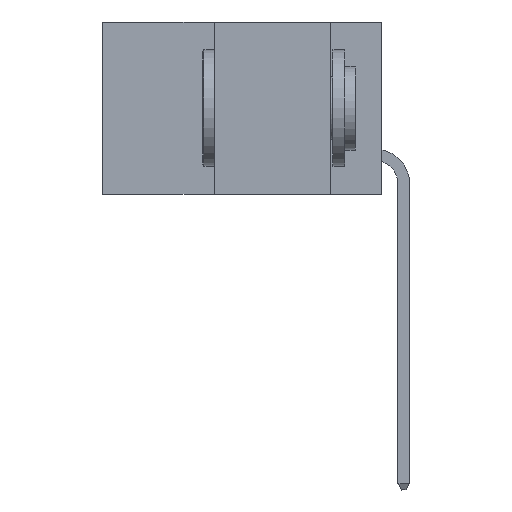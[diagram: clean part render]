
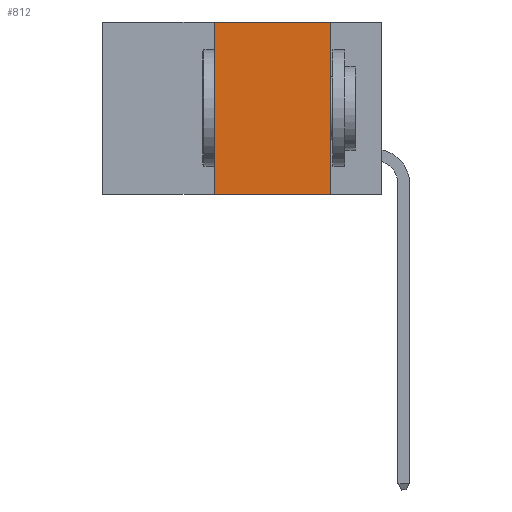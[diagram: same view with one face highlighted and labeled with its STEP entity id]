
A CAD part, left-side view. The second image highlights one B-rep face of the part: STEP entity #812.
In plain terms, the highlighted planar face has unit normal (-1, 0, 0).
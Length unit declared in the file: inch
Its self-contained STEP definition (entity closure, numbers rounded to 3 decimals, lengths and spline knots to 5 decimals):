
#757 = EDGE_CURVE ( 'NONE', #19557, #20888, #19914, .T. ) ;
#812 = ADVANCED_FACE ( 'NONE', ( #7493 ), #23499, .F. ) ;
#2360 = CARTESIAN_POINT ( 'NONE',  ( 0., 0.11, 0. ) ) ;
#3142 = EDGE_CURVE ( 'NONE', #5010, #19557, #9548, .T. ) ;
#3260 = CARTESIAN_POINT ( 'NONE',  ( 0., 0.6, 0. ) ) ;
#4250 = DIRECTION ( 'NONE',  ( 0., 0., -1. ) ) ;
#4699 = CARTESIAN_POINT ( 'NONE',  ( 0., 0.11, -0.37 ) ) ;
#5010 = VERTEX_POINT ( 'NONE', #23443 ) ;
#5250 = DIRECTION ( 'NONE',  ( 0., -1., 0. ) ) ;
#7194 = LINE ( 'NONE', #17725, #10431 ) ;
#7449 = ORIENTED_EDGE ( 'NONE', *, *, #3142, .F. ) ;
#7493 = FACE_OUTER_BOUND ( 'NONE', #8735, .T. ) ;
#8735 = EDGE_LOOP ( 'NONE', ( #23941, #7449, #8855, #21813 ) ) ;
#8855 = ORIENTED_EDGE ( 'NONE', *, *, #23285, .F. ) ;
#9548 = LINE ( 'NONE', #3260, #10712 ) ;
#9648 = CARTESIAN_POINT ( 'NONE',  ( 0., 0.36, 0. ) ) ;
#10431 = VECTOR ( 'NONE', #11960, 39.37008 ) ;
#10669 = CARTESIAN_POINT ( 'NONE',  ( 0., 0.36, -0.37 ) ) ;
#10712 = VECTOR ( 'NONE', #5250, 39.37008 ) ;
#11960 = DIRECTION ( 'NONE',  ( 0., -1., 0. ) ) ;
#13021 = VECTOR ( 'NONE', #18837, 39.37008 ) ;
#13977 = DIRECTION ( 'NONE',  ( 0., 0., -1. ) ) ;
#14029 = EDGE_CURVE ( 'NONE', #20859, #20888, #7194, .T. ) ;
#16403 = DIRECTION ( 'NONE',  ( 1., 0., 0. ) ) ;
#16799 = CARTESIAN_POINT ( 'NONE',  ( 0., 0.6, 0. ) ) ;
#17158 = CARTESIAN_POINT ( 'NONE',  ( 0., 0.11, 0. ) ) ;
#17725 = CARTESIAN_POINT ( 'NONE',  ( 0., 0.6, -0.37 ) ) ;
#18014 = LINE ( 'NONE', #9648, #13021 ) ;
#18837 = DIRECTION ( 'NONE',  ( 0., 0., 1. ) ) ;
#19557 = VERTEX_POINT ( 'NONE', #17158 ) ;
#19722 = AXIS2_PLACEMENT_3D ( 'NONE', #16799, #16403, #13977 ) ;
#19914 = LINE ( 'NONE', #2360, #21683 ) ;
#20859 = VERTEX_POINT ( 'NONE', #10669 ) ;
#20888 = VERTEX_POINT ( 'NONE', #4699 ) ;
#21683 = VECTOR ( 'NONE', #4250, 39.37008 ) ;
#21813 = ORIENTED_EDGE ( 'NONE', *, *, #14029, .T. ) ;
#23285 = EDGE_CURVE ( 'NONE', #20859, #5010, #18014, .T. ) ;
#23443 = CARTESIAN_POINT ( 'NONE',  ( 0., 0.36, 0. ) ) ;
#23499 = PLANE ( 'NONE',  #19722 ) ;
#23941 = ORIENTED_EDGE ( 'NONE', *, *, #757, .F. ) ;
